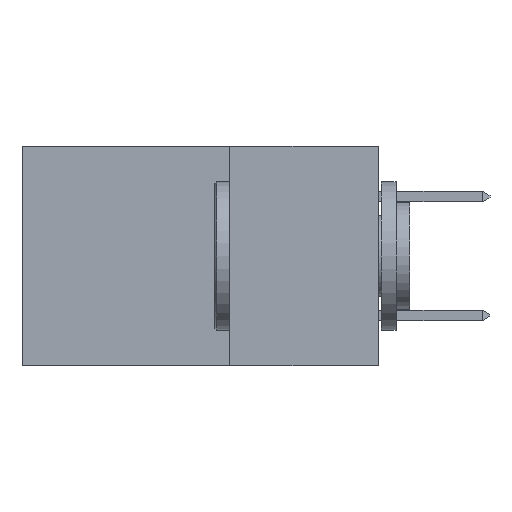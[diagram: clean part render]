
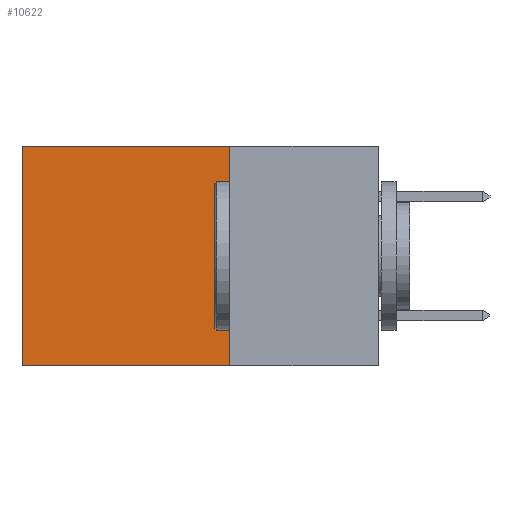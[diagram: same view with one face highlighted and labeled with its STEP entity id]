
A CAD part, left-side view. The second image highlights one B-rep face of the part: STEP entity #10622.
In plain terms, the highlighted planar face has unit normal (-1, 0, 0).
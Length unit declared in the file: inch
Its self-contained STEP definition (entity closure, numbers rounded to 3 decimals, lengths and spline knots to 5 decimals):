
#845 = DIRECTION ( 'NONE',  ( 0., 1., 0. ) ) ;
#854 = DIRECTION ( 'NONE',  ( 0., 1., 0. ) ) ;
#1170 = VERTEX_POINT ( 'NONE', #14007 ) ;
#1562 = VERTEX_POINT ( 'NONE', #13172 ) ;
#1580 = DIRECTION ( 'NONE',  ( 1., 0., 0. ) ) ;
#2015 = EDGE_CURVE ( 'NONE', #8203, #10258, #13853, .T. ) ;
#3508 = ORIENTED_EDGE ( 'NONE', *, *, #14894, .T. ) ;
#3733 = VECTOR ( 'NONE', #845, 39.37008 ) ;
#4667 = CARTESIAN_POINT ( 'NONE',  ( 0.298, 0.25, -0.37 ) ) ;
#4668 = VECTOR ( 'NONE', #12912, 39.37008 ) ;
#6966 = ORIENTED_EDGE ( 'NONE', *, *, #2015, .F. ) ;
#7022 = EDGE_LOOP ( 'NONE', ( #12815, #10368, #6966, #3508 ) ) ;
#7063 = CARTESIAN_POINT ( 'NONE',  ( 0.298, 0.25, 0. ) ) ;
#7082 = CARTESIAN_POINT ( 'NONE',  ( 0.298, 0.25, -0.37 ) ) ;
#7209 = LINE ( 'NONE', #14066, #13303 ) ;
#7308 = FACE_OUTER_BOUND ( 'NONE', #7022, .T. ) ;
#7697 = EDGE_CURVE ( 'NONE', #1170, #1562, #7209, .T. ) ;
#8203 = VERTEX_POINT ( 'NONE', #7063 ) ;
#8940 = CARTESIAN_POINT ( 'NONE',  ( 0.298, 0.25, 0. ) ) ;
#10101 = LINE ( 'NONE', #14950, #3733 ) ;
#10104 = DIRECTION ( 'NONE',  ( 0., 0., -1. ) ) ;
#10258 = VERTEX_POINT ( 'NONE', #7082 ) ;
#10368 = ORIENTED_EDGE ( 'NONE', *, *, #10807, .F. ) ;
#10622 = ADVANCED_FACE ( 'NONE', ( #7308 ), #12330, .F. ) ;
#10807 = EDGE_CURVE ( 'NONE', #10258, #1562, #11678, .T. ) ;
#10822 = DIRECTION ( 'NONE',  ( 0., 0., -1. ) ) ;
#10973 = VECTOR ( 'NONE', #854, 39.37008 ) ;
#11678 = LINE ( 'NONE', #4667, #10973 ) ;
#12330 = PLANE ( 'NONE',  #14745 ) ;
#12815 = ORIENTED_EDGE ( 'NONE', *, *, #7697, .T. ) ;
#12912 = DIRECTION ( 'NONE',  ( 0., 0., -1. ) ) ;
#13172 = CARTESIAN_POINT ( 'NONE',  ( 0.298, 0.6, -0.37 ) ) ;
#13303 = VECTOR ( 'NONE', #10822, 39.37008 ) ;
#13853 = LINE ( 'NONE', #14963, #4668 ) ;
#14007 = CARTESIAN_POINT ( 'NONE',  ( 0.298, 0.6, 0. ) ) ;
#14066 = CARTESIAN_POINT ( 'NONE',  ( 0.298, 0.6, 0. ) ) ;
#14745 = AXIS2_PLACEMENT_3D ( 'NONE', #8940, #1580, #10104 ) ;
#14894 = EDGE_CURVE ( 'NONE', #8203, #1170, #10101, .T. ) ;
#14950 = CARTESIAN_POINT ( 'NONE',  ( 0.298, 0.25, 0. ) ) ;
#14963 = CARTESIAN_POINT ( 'NONE',  ( 0.298, 0.25, 0. ) ) ;
